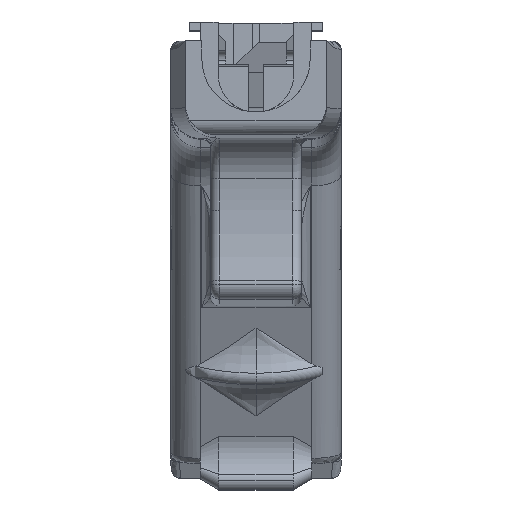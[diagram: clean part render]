
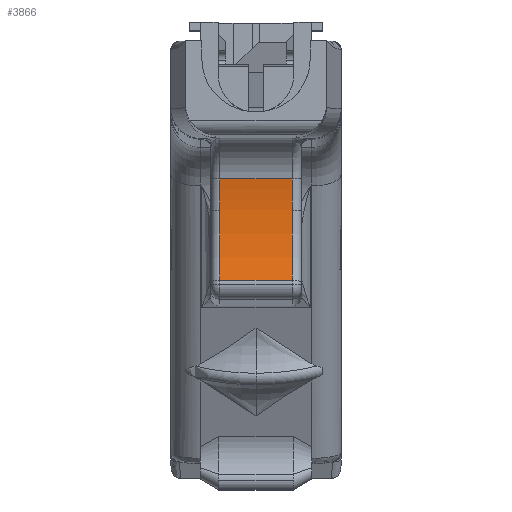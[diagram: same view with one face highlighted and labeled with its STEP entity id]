
A CAD part, top view. The second image highlights one B-rep face of the part: STEP entity #3866.
In plain terms, the highlighted cylindrical face has radius 41.155 mm (diameter 82.31 mm), a partial arc.
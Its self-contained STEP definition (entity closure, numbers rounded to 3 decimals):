
#32 = CARTESIAN_POINT ( 'NONE',  ( -6.223, -23.613, -39.936 ) ) ;
#40 = ORIENTED_EDGE ( 'NONE', *, *, #7833, .T. ) ;
#132 = ORIENTED_EDGE ( 'NONE', *, *, #4411, .T. ) ;
#226 = DIRECTION ( 'NONE',  ( 1., 0., 0. ) ) ;
#234 = DIRECTION ( 'NONE',  ( 0., 0., -1. ) ) ;
#430 = CIRCLE ( 'NONE', #2847, 41.155 ) ;
#1105 = EDGE_CURVE ( 'NONE', #4929, #4145, #430, .T. ) ;
#1125 = ORIENTED_EDGE ( 'NONE', *, *, #3308, .T. ) ;
#1128 = EDGE_CURVE ( 'NONE', #4956, #5690, #5826, .T. ) ;
#1215 = EDGE_LOOP ( 'NONE', ( #132, #3453, #1125, #5055, #2528, #40 ) ) ;
#1496 = AXIS2_PLACEMENT_3D ( 'NONE', #10358, #4295, #11391 ) ;
#2057 = LINE ( 'NONE', #12882, #12540 ) ;
#2528 = ORIENTED_EDGE ( 'NONE', *, *, #1128, .T. ) ;
#2847 = AXIS2_PLACEMENT_3D ( 'NONE', #12367, #6304, #234 ) ;
#3308 = EDGE_CURVE ( 'NONE', #4145, #5095, #13074, .T. ) ;
#3334 = DIRECTION ( 'NONE',  ( -1., 0., 0. ) ) ;
#3453 = ORIENTED_EDGE ( 'NONE', *, *, #1105, .T. ) ;
#3866 = ADVANCED_FACE ( 'NONE', ( #5299 ), #13062, .F. ) ;
#4145 = VERTEX_POINT ( 'NONE', #5817 ) ;
#4171 = CARTESIAN_POINT ( 'NONE',  ( -6.223, -40.969, -38.514 ) ) ;
#4295 = DIRECTION ( 'NONE',  ( 1., 0., 0. ) ) ;
#4411 = EDGE_CURVE ( 'NONE', #11330, #4929, #12287, .T. ) ;
#4431 = AXIS2_PLACEMENT_3D ( 'NONE', #9435, #3334, #10436 ) ;
#4550 = CARTESIAN_POINT ( 'NONE',  ( 6.223, -29.007, -40.291 ) ) ;
#4841 = VECTOR ( 'NONE', #5270, 1000. ) ;
#4929 = VERTEX_POINT ( 'NONE', #32 ) ;
#4956 = VERTEX_POINT ( 'NONE', #12198 ) ;
#4966 = AXIS2_PLACEMENT_3D ( 'NONE', #6290, #226, #7324 ) ;
#5055 = ORIENTED_EDGE ( 'NONE', *, *, #7237, .F. ) ;
#5095 = VERTEX_POINT ( 'NONE', #4171 ) ;
#5148 = CARTESIAN_POINT ( 'NONE',  ( 7.747, -29.007, 0.864 ) ) ;
#5270 = DIRECTION ( 'NONE',  ( -1., 0., 0. ) ) ;
#5299 = FACE_OUTER_BOUND ( 'NONE', #1215, .T. ) ;
#5690 = VERTEX_POINT ( 'NONE', #4550 ) ;
#5817 = CARTESIAN_POINT ( 'NONE',  ( -6.223, -29.007, -40.291 ) ) ;
#5826 = CIRCLE ( 'NONE', #1496, 41.155 ) ;
#6215 = DIRECTION ( 'NONE',  ( -1., 0., 0. ) ) ;
#6290 = CARTESIAN_POINT ( 'NONE',  ( 6.223, -29.007, 0.864 ) ) ;
#6304 = DIRECTION ( 'NONE',  ( -1., 0., 0. ) ) ;
#6823 = DIRECTION ( 'NONE',  ( -1., 0., 0. ) ) ;
#7237 = EDGE_CURVE ( 'NONE', #4956, #5095, #2057, .T. ) ;
#7324 = DIRECTION ( 'NONE',  ( 0., 0., -1. ) ) ;
#7833 = EDGE_CURVE ( 'NONE', #5690, #11330, #8109, .T. ) ;
#8109 = CIRCLE ( 'NONE', #4966, 41.155 ) ;
#8171 = DIRECTION ( 'NONE',  ( 0., 0., 1. ) ) ;
#9435 = CARTESIAN_POINT ( 'NONE',  ( -6.223, -29.007, 0.864 ) ) ;
#10358 = CARTESIAN_POINT ( 'NONE',  ( 6.223, -29.007, 0.864 ) ) ;
#10436 = DIRECTION ( 'NONE',  ( 0., 0., -1. ) ) ;
#11330 = VERTEX_POINT ( 'NONE', #11508 ) ;
#11333 = CARTESIAN_POINT ( 'NONE',  ( 7.747, -23.613, -39.936 ) ) ;
#11391 = DIRECTION ( 'NONE',  ( 0., 0., -1. ) ) ;
#11508 = CARTESIAN_POINT ( 'NONE',  ( 6.223, -23.613, -39.936 ) ) ;
#12198 = CARTESIAN_POINT ( 'NONE',  ( 6.223, -40.969, -38.514 ) ) ;
#12287 = LINE ( 'NONE', #11333, #4841 ) ;
#12367 = CARTESIAN_POINT ( 'NONE',  ( -6.223, -29.007, 0.864 ) ) ;
#12540 = VECTOR ( 'NONE', #6823, 1000. ) ;
#12757 = AXIS2_PLACEMENT_3D ( 'NONE', #5148, #6215, #8171 ) ;
#12882 = CARTESIAN_POINT ( 'NONE',  ( 7.747, -40.969, -38.514 ) ) ;
#13062 = CYLINDRICAL_SURFACE ( 'NONE', #12757, 41.155 ) ;
#13074 = CIRCLE ( 'NONE', #4431, 41.155 ) ;
